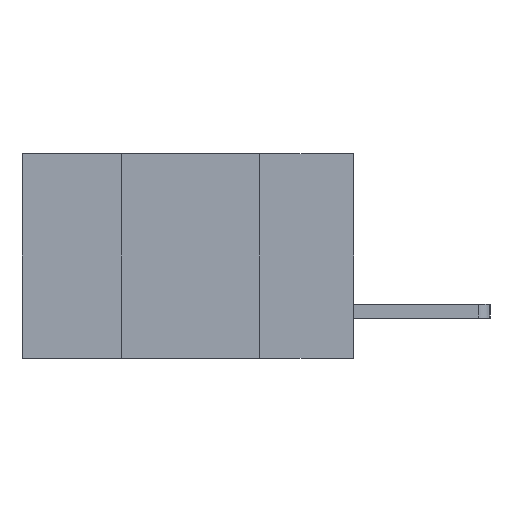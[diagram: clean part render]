
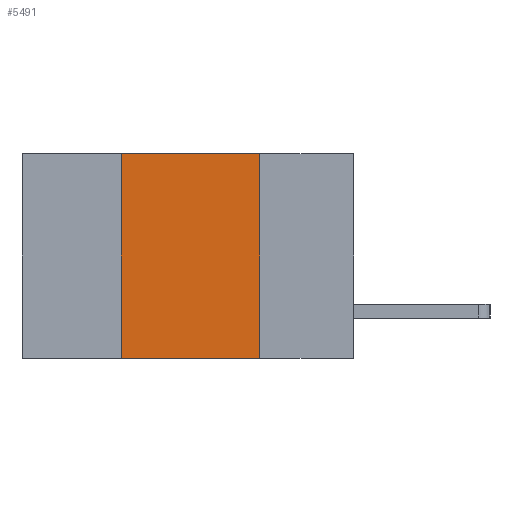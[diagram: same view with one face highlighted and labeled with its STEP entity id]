
A CAD part, left-side view. The second image highlights one B-rep face of the part: STEP entity #5491.
In plain terms, the highlighted planar face has unit normal (-1, 0, 0).
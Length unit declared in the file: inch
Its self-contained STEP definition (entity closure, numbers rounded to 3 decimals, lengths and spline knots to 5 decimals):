
#86 = CARTESIAN_POINT ( 'NONE',  ( 0., 0.17, 0. ) ) ;
#214 = CARTESIAN_POINT ( 'NONE',  ( 0., 0.6, -0.37 ) ) ;
#316 = LINE ( 'NONE', #86, #7176 ) ;
#555 = AXIS2_PLACEMENT_3D ( 'NONE', #3437, #2662, #2487 ) ;
#1372 = CARTESIAN_POINT ( 'NONE',  ( 0., 0.17, -0.37 ) ) ;
#1563 = PLANE ( 'NONE',  #555 ) ;
#1671 = EDGE_LOOP ( 'NONE', ( #10917, #8312, #11532, #2468 ) ) ;
#1767 = CARTESIAN_POINT ( 'NONE',  ( 0., 0.6, 0. ) ) ;
#2468 = ORIENTED_EDGE ( 'NONE', *, *, #7319, .T. ) ;
#2487 = DIRECTION ( 'NONE',  ( 0., 0., -1. ) ) ;
#2662 = DIRECTION ( 'NONE',  ( 1., 0., 0. ) ) ;
#3087 = EDGE_CURVE ( 'NONE', #5757, #11638, #5295, .T. ) ;
#3209 = EDGE_CURVE ( 'NONE', #7024, #5757, #10716, .T. ) ;
#3437 = CARTESIAN_POINT ( 'NONE',  ( 0., 0.6, 0. ) ) ;
#3624 = DIRECTION ( 'NONE',  ( 0., -1., 0. ) ) ;
#4811 = VECTOR ( 'NONE', #7459, 39.37008 ) ;
#5156 = CARTESIAN_POINT ( 'NONE',  ( 0., 0.42, 0. ) ) ;
#5295 = LINE ( 'NONE', #1767, #8628 ) ;
#5491 = ADVANCED_FACE ( 'NONE', ( #10957 ), #1563, .F. ) ;
#5757 = VERTEX_POINT ( 'NONE', #7831 ) ;
#6096 = CARTESIAN_POINT ( 'NONE',  ( 0., 0.17, 0. ) ) ;
#7024 = VERTEX_POINT ( 'NONE', #10589 ) ;
#7086 = VERTEX_POINT ( 'NONE', #1372 ) ;
#7176 = VECTOR ( 'NONE', #8587, 39.37008 ) ;
#7319 = EDGE_CURVE ( 'NONE', #7024, #7086, #8487, .T. ) ;
#7459 = DIRECTION ( 'NONE',  ( 0., -1., 0. ) ) ;
#7831 = CARTESIAN_POINT ( 'NONE',  ( 0., 0.42, 0. ) ) ;
#8312 = ORIENTED_EDGE ( 'NONE', *, *, #3087, .F. ) ;
#8487 = LINE ( 'NONE', #214, #4811 ) ;
#8587 = DIRECTION ( 'NONE',  ( 0., 0., -1. ) ) ;
#8628 = VECTOR ( 'NONE', #3624, 39.37008 ) ;
#8869 = DIRECTION ( 'NONE',  ( 0., 0., 1. ) ) ;
#8962 = EDGE_CURVE ( 'NONE', #11638, #7086, #316, .T. ) ;
#9761 = VECTOR ( 'NONE', #8869, 39.37008 ) ;
#10589 = CARTESIAN_POINT ( 'NONE',  ( 0., 0.42, -0.37 ) ) ;
#10716 = LINE ( 'NONE', #5156, #9761 ) ;
#10917 = ORIENTED_EDGE ( 'NONE', *, *, #8962, .F. ) ;
#10957 = FACE_OUTER_BOUND ( 'NONE', #1671, .T. ) ;
#11532 = ORIENTED_EDGE ( 'NONE', *, *, #3209, .F. ) ;
#11638 = VERTEX_POINT ( 'NONE', #6096 ) ;
